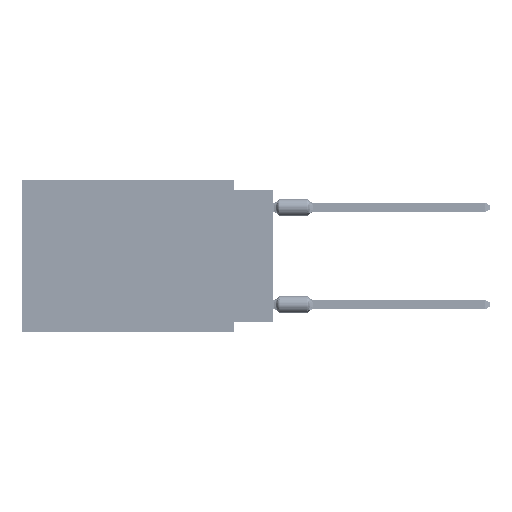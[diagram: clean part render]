
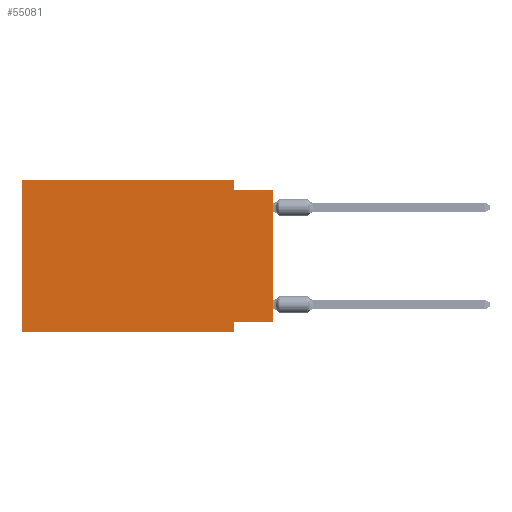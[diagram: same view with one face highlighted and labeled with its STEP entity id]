
A CAD part, left-side view. The second image highlights one B-rep face of the part: STEP entity #55081.
In plain terms, the highlighted planar face has unit normal (-1, 0, 0).
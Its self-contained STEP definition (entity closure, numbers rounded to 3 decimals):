
#446 = EDGE_CURVE ( 'NONE', #6810, #47571, #74948, .T. ) ;
#845 = VECTOR ( 'NONE', #39217, 1000. ) ;
#894 = EDGE_CURVE ( 'NONE', #70440, #3131, #52887, .T. ) ;
#3131 = VERTEX_POINT ( 'NONE', #45554 ) ;
#4696 = DIRECTION ( 'NONE',  ( 0., 0., -1. ) ) ;
#6810 = VERTEX_POINT ( 'NONE', #71008 ) ;
#7366 = CARTESIAN_POINT ( 'NONE',  ( 0., 2.54, -9.906 ) ) ;
#11028 = ORIENTED_EDGE ( 'NONE', *, *, #22805, .F. ) ;
#11046 = FACE_OUTER_BOUND ( 'NONE', #84947, .T. ) ;
#11709 = EDGE_CURVE ( 'NONE', #53229, #82035, #78760, .T. ) ;
#13860 = EDGE_CURVE ( 'NONE', #6810, #18384, #86332, .T. ) ;
#15849 = LINE ( 'NONE', #79622, #39033 ) ;
#18384 = VERTEX_POINT ( 'NONE', #61805 ) ;
#18721 = ORIENTED_EDGE ( 'NONE', *, *, #28259, .F. ) ;
#21924 = AXIS2_PLACEMENT_3D ( 'NONE', #67125, #80781, #4696 ) ;
#22805 = EDGE_CURVE ( 'NONE', #53229, #77990, #15849, .T. ) ;
#23149 = DIRECTION ( 'NONE',  ( 0., 0., 1. ) ) ;
#23893 = DIRECTION ( 'NONE',  ( 0., 0., 1. ) ) ;
#28259 = EDGE_CURVE ( 'NONE', #3131, #82035, #76383, .T. ) ;
#28416 = VECTOR ( 'NONE', #32592, 1000. ) ;
#29199 = EDGE_CURVE ( 'NONE', #77990, #47571, #83028, .T. ) ;
#29247 = DIRECTION ( 'NONE',  ( 0., 0., -1. ) ) ;
#29987 = CARTESIAN_POINT ( 'NONE',  ( 0., 0., 0. ) ) ;
#32592 = DIRECTION ( 'NONE',  ( 0., -1., 0. ) ) ;
#36872 = VECTOR ( 'NONE', #84124, 1000. ) ;
#37121 = CARTESIAN_POINT ( 'NONE',  ( 0., 16.383, 0. ) ) ;
#39033 = VECTOR ( 'NONE', #86440, 1000. ) ;
#39217 = DIRECTION ( 'NONE',  ( 0., 0., -1. ) ) ;
#41017 = LINE ( 'NONE', #68813, #63656 ) ;
#41747 = CARTESIAN_POINT ( 'NONE',  ( 0., 0., -0.635 ) ) ;
#44105 = VECTOR ( 'NONE', #23149, 1000. ) ;
#45554 = CARTESIAN_POINT ( 'NONE',  ( 0., 2.54, -0.635 ) ) ;
#46135 = PLANE ( 'NONE',  #21924 ) ;
#46265 = CARTESIAN_POINT ( 'NONE',  ( 0., 16.383, -9.906 ) ) ;
#47571 = VERTEX_POINT ( 'NONE', #52805 ) ;
#49198 = CARTESIAN_POINT ( 'NONE',  ( 0., 0., -9.271 ) ) ;
#52805 = CARTESIAN_POINT ( 'NONE',  ( 0., 2.54, -9.906 ) ) ;
#52887 = LINE ( 'NONE', #75186, #845 ) ;
#53229 = VERTEX_POINT ( 'NONE', #49198 ) ;
#55024 = ORIENTED_EDGE ( 'NONE', *, *, #13860, .F. ) ;
#55081 = ADVANCED_FACE ( 'NONE', ( #11046 ), #46135, .F. ) ;
#57127 = CARTESIAN_POINT ( 'NONE',  ( 0., 2.54, -9.271 ) ) ;
#58490 = ORIENTED_EDGE ( 'NONE', *, *, #446, .T. ) ;
#61546 = ORIENTED_EDGE ( 'NONE', *, *, #29199, .F. ) ;
#61805 = CARTESIAN_POINT ( 'NONE',  ( 0., 16.383, 0. ) ) ;
#63656 = VECTOR ( 'NONE', #89752, 1000. ) ;
#67125 = CARTESIAN_POINT ( 'NONE',  ( 0., 16.383, 0. ) ) ;
#68813 = CARTESIAN_POINT ( 'NONE',  ( 0., 16.383, 0. ) ) ;
#70440 = VERTEX_POINT ( 'NONE', #86428 ) ;
#71008 = CARTESIAN_POINT ( 'NONE',  ( 0., 16.383, -9.906 ) ) ;
#72744 = ORIENTED_EDGE ( 'NONE', *, *, #11709, .T. ) ;
#74948 = LINE ( 'NONE', #46265, #28416 ) ;
#75046 = ORIENTED_EDGE ( 'NONE', *, *, #894, .F. ) ;
#75186 = CARTESIAN_POINT ( 'NONE',  ( 0., 2.54, 0. ) ) ;
#76383 = LINE ( 'NONE', #41747, #36872 ) ;
#76766 = ORIENTED_EDGE ( 'NONE', *, *, #84359, .F. ) ;
#77990 = VERTEX_POINT ( 'NONE', #57127 ) ;
#78760 = LINE ( 'NONE', #29987, #44105 ) ;
#79622 = CARTESIAN_POINT ( 'NONE',  ( 0., 0., -9.271 ) ) ;
#80781 = DIRECTION ( 'NONE',  ( 1., 0., 0. ) ) ;
#82035 = VERTEX_POINT ( 'NONE', #84236 ) ;
#83028 = LINE ( 'NONE', #7366, #83735 ) ;
#83735 = VECTOR ( 'NONE', #29247, 1000. ) ;
#84124 = DIRECTION ( 'NONE',  ( 0., -1., 0. ) ) ;
#84236 = CARTESIAN_POINT ( 'NONE',  ( 0., 0., -0.635 ) ) ;
#84359 = EDGE_CURVE ( 'NONE', #18384, #70440, #41017, .T. ) ;
#84947 = EDGE_LOOP ( 'NONE', ( #72744, #18721, #75046, #76766, #55024, #58490, #61546, #11028 ) ) ;
#86230 = VECTOR ( 'NONE', #23893, 1000. ) ;
#86332 = LINE ( 'NONE', #37121, #86230 ) ;
#86428 = CARTESIAN_POINT ( 'NONE',  ( 0., 2.54, 0. ) ) ;
#86440 = DIRECTION ( 'NONE',  ( 0., 1., 0. ) ) ;
#89752 = DIRECTION ( 'NONE',  ( 0., -1., 0. ) ) ;
